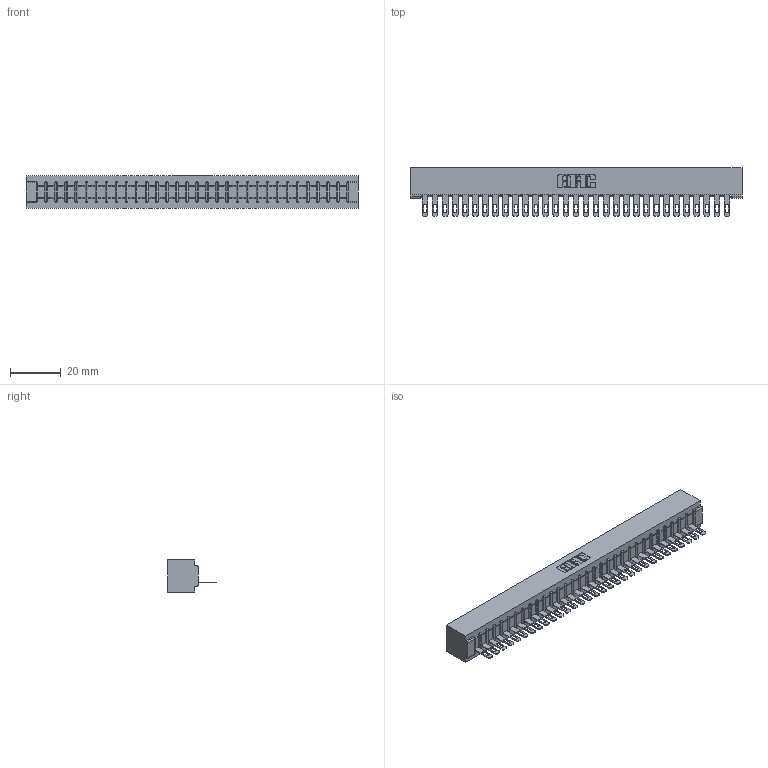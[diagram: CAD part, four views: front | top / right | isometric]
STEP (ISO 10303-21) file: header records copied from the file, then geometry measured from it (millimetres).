
FILE_DESCRIPTION (( 'STEP AP203' ), '1' );
FILE_NAME ('307-031-505-101.STEP', '2019-09-04T00:16:18', ( '' ), ( '' ), 'SwSTEP 2.0', 'SolidWorks 2016', '' );
FILE_SCHEMA (( 'CONFIG_CONTROL_DESIGN' ));
Length unit declared in the file: inch
Products named in the file (3): 307-031-505-101; 307 Part_No Mounting Lugs; 307-290-001_505
Assembly tree (32 placements, depth 2):
  307-031-505-101
    307 Part_No Mounting Lugs
    307-290-001_505  x31
Bounding box: 130.71 x 19.18 x 12.7 mm (x, y, z)
Volume: 14057.7 mm3; surface area: 15161 mm2
Topology: 32 solids, 32 shells, 1878 faces, 5321 edges, 3418 vertices
Faces by surface type: plane 1182, cylinder 632, sphere 64
Entity records: 27628 total; most frequent: CARTESIAN_POINT 4648, ORIENTED_EDGE 4634, DIRECTION 4527, EDGE_CURVE 2317, LINE 1773, VECTOR 1773, VERTEX_POINT 1498, AXIS2_PLACEMENT_3D 1377
